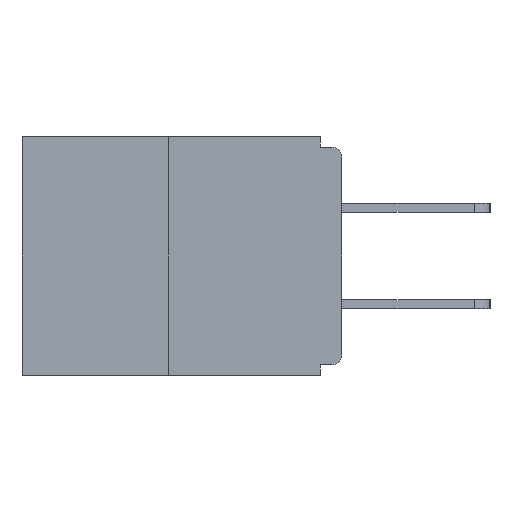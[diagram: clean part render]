
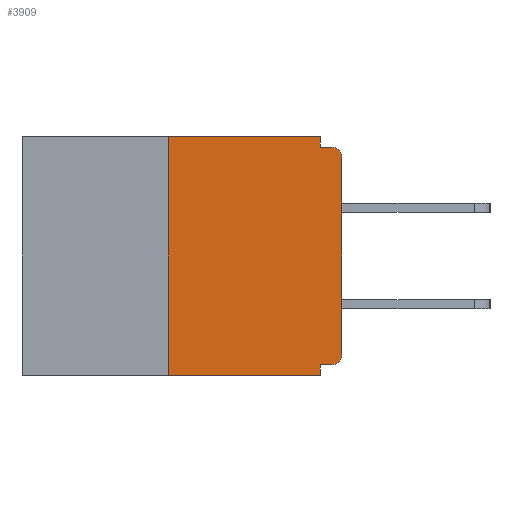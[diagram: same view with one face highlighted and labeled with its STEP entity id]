
A CAD part, left-side view. The second image highlights one B-rep face of the part: STEP entity #3909.
In plain terms, the highlighted planar face has unit normal (-1, 0, 0).
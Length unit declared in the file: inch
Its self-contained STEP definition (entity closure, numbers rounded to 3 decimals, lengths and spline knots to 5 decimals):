
#69 = LINE ( 'NONE', #11062, #14020 ) ;
#340 = CARTESIAN_POINT ( 'NONE',  ( 0., 0., -0.03 ) ) ;
#566 = VERTEX_POINT ( 'NONE', #9889 ) ;
#646 = DIRECTION ( 'NONE',  ( 0., 0., 1. ) ) ;
#737 = AXIS2_PLACEMENT_3D ( 'NONE', #6702, #9466, #10921 ) ;
#1026 = LINE ( 'NONE', #10882, #14988 ) ;
#1056 = DIRECTION ( 'NONE',  ( 0., -1., 0. ) ) ;
#1063 = CARTESIAN_POINT ( 'NONE',  ( 0., 0.25, -0.343 ) ) ;
#1455 = LINE ( 'NONE', #10293, #14748 ) ;
#1546 = CARTESIAN_POINT ( 'NONE',  ( 0., 0.25, 0. ) ) ;
#1567 = CARTESIAN_POINT ( 'NONE',  ( 0., 0.031, -0.343 ) ) ;
#1935 = EDGE_CURVE ( 'NONE', #18624, #12863, #9054, .T. ) ;
#2372 = AXIS2_PLACEMENT_3D ( 'NONE', #17318, #9980, #10701 ) ;
#2709 = CARTESIAN_POINT ( 'NONE',  ( 0., 0.015, -0.328 ) ) ;
#2868 = CIRCLE ( 'NONE', #2372, 0.015 ) ;
#2979 = ORIENTED_EDGE ( 'NONE', *, *, #7014, .F. ) ;
#3066 = LINE ( 'NONE', #10768, #5526 ) ;
#3195 = VERTEX_POINT ( 'NONE', #17020 ) ;
#3385 = VERTEX_POINT ( 'NONE', #1567 ) ;
#3909 = ADVANCED_FACE ( 'NONE', ( #5437 ), #5420, .F. ) ;
#4007 = VECTOR ( 'NONE', #16711, 39.37008 ) ;
#4403 = CARTESIAN_POINT ( 'NONE',  ( 0., 0., 0. ) ) ;
#5200 = VERTEX_POINT ( 'NONE', #2709 ) ;
#5361 = CARTESIAN_POINT ( 'NONE',  ( 0., 0.031, -0.328 ) ) ;
#5404 = DIRECTION ( 'NONE',  ( 0., 0., 1. ) ) ;
#5420 = PLANE ( 'NONE',  #16501 ) ;
#5437 = FACE_OUTER_BOUND ( 'NONE', #13262, .T. ) ;
#5475 = DIRECTION ( 'NONE',  ( 0., 0., -1. ) ) ;
#5526 = VECTOR ( 'NONE', #646, 39.37008 ) ;
#6702 = CARTESIAN_POINT ( 'NONE',  ( 0., 0.015, -0.03 ) ) ;
#7014 = EDGE_CURVE ( 'NONE', #12583, #3385, #1455, .T. ) ;
#7030 = LINE ( 'NONE', #9658, #4007 ) ;
#7498 = ORIENTED_EDGE ( 'NONE', *, *, #12592, .T. ) ;
#7613 = CIRCLE ( 'NONE', #737, 0.015 ) ;
#7753 = DIRECTION ( 'NONE',  ( 0., 0., -1. ) ) ;
#8555 = EDGE_CURVE ( 'NONE', #3195, #17629, #69, .T. ) ;
#8816 = ORIENTED_EDGE ( 'NONE', *, *, #18426, .T. ) ;
#9054 = LINE ( 'NONE', #15474, #11939 ) ;
#9381 = ORIENTED_EDGE ( 'NONE', *, *, #14284, .F. ) ;
#9459 = ORIENTED_EDGE ( 'NONE', *, *, #1935, .F. ) ;
#9466 = DIRECTION ( 'NONE',  ( -1., 0., 0. ) ) ;
#9658 = CARTESIAN_POINT ( 'NONE',  ( 0., 0., -0.328 ) ) ;
#9732 = CARTESIAN_POINT ( 'NONE',  ( 0., 0.031, 0. ) ) ;
#9773 = ORIENTED_EDGE ( 'NONE', *, *, #11667, .T. ) ;
#9823 = LINE ( 'NONE', #4403, #11816 ) ;
#9889 = CARTESIAN_POINT ( 'NONE',  ( 0., 0., -0.313 ) ) ;
#9980 = DIRECTION ( 'NONE',  ( -1., 0., 0. ) ) ;
#10293 = CARTESIAN_POINT ( 'NONE',  ( 0., 0.031, -0.343 ) ) ;
#10701 = DIRECTION ( 'NONE',  ( 0., 0., -1. ) ) ;
#10768 = CARTESIAN_POINT ( 'NONE',  ( 0., 0.25, 0. ) ) ;
#10882 = CARTESIAN_POINT ( 'NONE',  ( 0., 0.46, -0.343 ) ) ;
#10921 = DIRECTION ( 'NONE',  ( 0., 0., -1. ) ) ;
#11062 = CARTESIAN_POINT ( 'NONE',  ( 0., 0., -0.015 ) ) ;
#11201 = VERTEX_POINT ( 'NONE', #340 ) ;
#11666 = ORIENTED_EDGE ( 'NONE', *, *, #18453, .F. ) ;
#11667 = EDGE_CURVE ( 'NONE', #5200, #566, #2868, .T. ) ;
#11775 = ORIENTED_EDGE ( 'NONE', *, *, #18128, .T. ) ;
#11816 = VECTOR ( 'NONE', #5404, 39.37008 ) ;
#11939 = VECTOR ( 'NONE', #16990, 39.37008 ) ;
#12325 = DIRECTION ( 'NONE',  ( 0., -1., 0. ) ) ;
#12583 = VERTEX_POINT ( 'NONE', #5361 ) ;
#12592 = EDGE_CURVE ( 'NONE', #13162, #3385, #1026, .T. ) ;
#12863 = VERTEX_POINT ( 'NONE', #9732 ) ;
#13055 = EDGE_CURVE ( 'NONE', #13162, #18624, #3066, .T. ) ;
#13162 = VERTEX_POINT ( 'NONE', #1063 ) ;
#13193 = DIRECTION ( 'NONE',  ( 0., 0., -1. ) ) ;
#13262 = EDGE_LOOP ( 'NONE', ( #9459, #17748, #7498, #2979, #11666, #9773, #11775, #8816, #16159, #9381 ) ) ;
#13702 = CARTESIAN_POINT ( 'NONE',  ( 0., 0.015, -0.015 ) ) ;
#13973 = DIRECTION ( 'NONE',  ( 1., 0., 0. ) ) ;
#14020 = VECTOR ( 'NONE', #1056, 39.37008 ) ;
#14109 = CARTESIAN_POINT ( 'NONE',  ( 0., 0.46, 0. ) ) ;
#14284 = EDGE_CURVE ( 'NONE', #12863, #3195, #16512, .T. ) ;
#14748 = VECTOR ( 'NONE', #13193, 39.37008 ) ;
#14988 = VECTOR ( 'NONE', #12325, 39.37008 ) ;
#15474 = CARTESIAN_POINT ( 'NONE',  ( 0., 0.46, 0. ) ) ;
#16159 = ORIENTED_EDGE ( 'NONE', *, *, #8555, .F. ) ;
#16501 = AXIS2_PLACEMENT_3D ( 'NONE', #14109, #13973, #5475 ) ;
#16512 = LINE ( 'NONE', #17799, #18105 ) ;
#16711 = DIRECTION ( 'NONE',  ( 0., 1., 0. ) ) ;
#16990 = DIRECTION ( 'NONE',  ( 0., -1., 0. ) ) ;
#17020 = CARTESIAN_POINT ( 'NONE',  ( 0., 0.031, -0.015 ) ) ;
#17318 = CARTESIAN_POINT ( 'NONE',  ( 0., 0.015, -0.313 ) ) ;
#17629 = VERTEX_POINT ( 'NONE', #13702 ) ;
#17748 = ORIENTED_EDGE ( 'NONE', *, *, #13055, .F. ) ;
#17799 = CARTESIAN_POINT ( 'NONE',  ( 0., 0.031, 0. ) ) ;
#18105 = VECTOR ( 'NONE', #7753, 39.37008 ) ;
#18128 = EDGE_CURVE ( 'NONE', #566, #11201, #9823, .T. ) ;
#18426 = EDGE_CURVE ( 'NONE', #11201, #17629, #7613, .T. ) ;
#18453 = EDGE_CURVE ( 'NONE', #5200, #12583, #7030, .T. ) ;
#18624 = VERTEX_POINT ( 'NONE', #1546 ) ;
